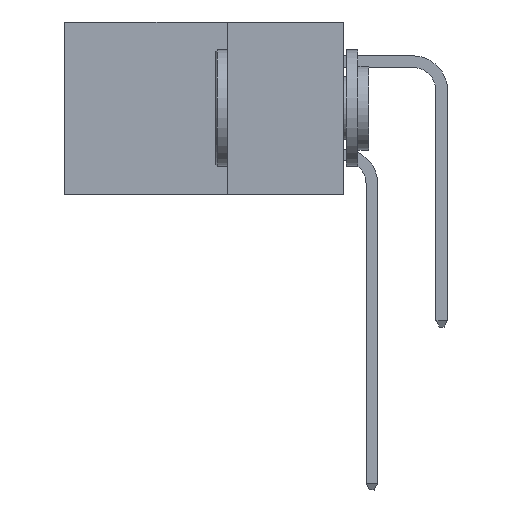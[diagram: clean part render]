
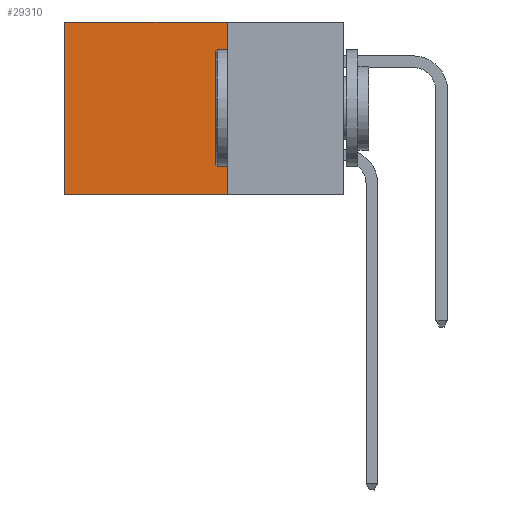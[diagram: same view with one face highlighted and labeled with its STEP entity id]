
A CAD part, left-side view. The second image highlights one B-rep face of the part: STEP entity #29310.
In plain terms, the highlighted planar face has unit normal (-1, 0, 0).
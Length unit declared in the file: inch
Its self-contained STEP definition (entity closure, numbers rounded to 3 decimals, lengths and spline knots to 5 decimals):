
#396 = DIRECTION ( 'NONE',  ( 0., 0., -1. ) ) ;
#954 = VERTEX_POINT ( 'NONE', #26368 ) ;
#1233 = VECTOR ( 'NONE', #10369, 39.37008 ) ;
#1268 = ORIENTED_EDGE ( 'NONE', *, *, #23348, .F. ) ;
#2263 = VECTOR ( 'NONE', #16219, 39.37008 ) ;
#2911 = CARTESIAN_POINT ( 'NONE',  ( 0.298, 0.6, 0. ) ) ;
#3735 = DIRECTION ( 'NONE',  ( 0., 0., -1. ) ) ;
#5704 = LINE ( 'NONE', #6795, #12502 ) ;
#5917 = EDGE_CURVE ( 'NONE', #29657, #17498, #14011, .T. ) ;
#6246 = CARTESIAN_POINT ( 'NONE',  ( 0.298, 0.25, 0. ) ) ;
#6795 = CARTESIAN_POINT ( 'NONE',  ( 0.298, 0.25, -0.37 ) ) ;
#7366 = LINE ( 'NONE', #17251, #1233 ) ;
#7878 = CARTESIAN_POINT ( 'NONE',  ( 0.298, 0.25, 0. ) ) ;
#7909 = VECTOR ( 'NONE', #396, 39.37008 ) ;
#8343 = DIRECTION ( 'NONE',  ( 1., 0., 0. ) ) ;
#9093 = ORIENTED_EDGE ( 'NONE', *, *, #19275, .T. ) ;
#10369 = DIRECTION ( 'NONE',  ( 0., 1., 0. ) ) ;
#12502 = VECTOR ( 'NONE', #13705, 39.37008 ) ;
#13705 = DIRECTION ( 'NONE',  ( 0., 1., 0. ) ) ;
#13737 = EDGE_CURVE ( 'NONE', #24157, #954, #14475, .T. ) ;
#14011 = LINE ( 'NONE', #2911, #7909 ) ;
#14270 = ORIENTED_EDGE ( 'NONE', *, *, #5917, .T. ) ;
#14475 = LINE ( 'NONE', #7878, #2263 ) ;
#16219 = DIRECTION ( 'NONE',  ( 0., 0., -1. ) ) ;
#17251 = CARTESIAN_POINT ( 'NONE',  ( 0.298, 0.25, 0. ) ) ;
#17498 = VERTEX_POINT ( 'NONE', #26548 ) ;
#19275 = EDGE_CURVE ( 'NONE', #24157, #29657, #7366, .T. ) ;
#21685 = ORIENTED_EDGE ( 'NONE', *, *, #13737, .F. ) ;
#22179 = PLANE ( 'NONE',  #29774 ) ;
#23348 = EDGE_CURVE ( 'NONE', #954, #17498, #5704, .T. ) ;
#24157 = VERTEX_POINT ( 'NONE', #25410 ) ;
#25410 = CARTESIAN_POINT ( 'NONE',  ( 0.298, 0.25, 0. ) ) ;
#25893 = FACE_OUTER_BOUND ( 'NONE', #27314, .T. ) ;
#26368 = CARTESIAN_POINT ( 'NONE',  ( 0.298, 0.25, -0.37 ) ) ;
#26548 = CARTESIAN_POINT ( 'NONE',  ( 0.298, 0.6, -0.37 ) ) ;
#27314 = EDGE_LOOP ( 'NONE', ( #14270, #1268, #21685, #9093 ) ) ;
#27999 = CARTESIAN_POINT ( 'NONE',  ( 0.298, 0.6, 0. ) ) ;
#29310 = ADVANCED_FACE ( 'NONE', ( #25893 ), #22179, .F. ) ;
#29657 = VERTEX_POINT ( 'NONE', #27999 ) ;
#29774 = AXIS2_PLACEMENT_3D ( 'NONE', #6246, #8343, #3735 ) ;
